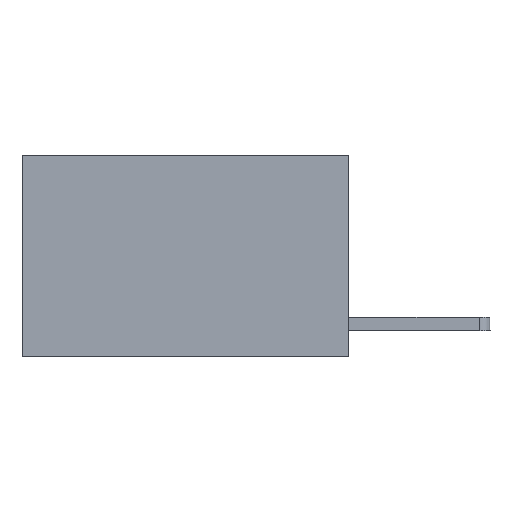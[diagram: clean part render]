
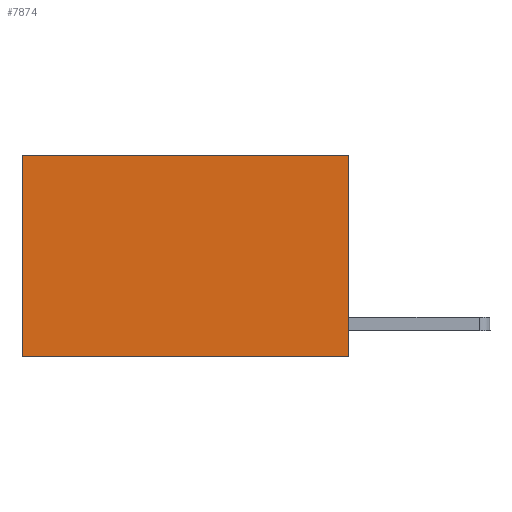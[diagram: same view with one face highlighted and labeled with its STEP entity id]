
A CAD part, left-side view. The second image highlights one B-rep face of the part: STEP entity #7874.
In plain terms, the highlighted planar face has unit normal (-1, 0, 0).
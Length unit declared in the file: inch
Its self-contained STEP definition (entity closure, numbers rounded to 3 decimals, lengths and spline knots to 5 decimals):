
#74 = EDGE_CURVE ( 'NONE', #4193, #2986, #7258, .T. ) ;
#390 = DIRECTION ( 'NONE',  ( 0., 1., 0. ) ) ;
#688 = CARTESIAN_POINT ( 'NONE',  ( 0.2625, 0., 0. ) ) ;
#774 = DIRECTION ( 'NONE',  ( 0., 0., -1. ) ) ;
#802 = DIRECTION ( 'NONE',  ( 0., 0., -1. ) ) ;
#911 = VECTOR ( 'NONE', #802, 39.37008 ) ;
#1186 = CARTESIAN_POINT ( 'NONE',  ( 0.2625, 0., -0.37 ) ) ;
#1474 = CARTESIAN_POINT ( 'NONE',  ( 0.2625, 0., 0. ) ) ;
#1542 = EDGE_LOOP ( 'NONE', ( #5234, #8449, #3500, #1996 ) ) ;
#1859 = EDGE_CURVE ( 'NONE', #2853, #7615, #8200, .T. ) ;
#1996 = ORIENTED_EDGE ( 'NONE', *, *, #3103, .T. ) ;
#2069 = AXIS2_PLACEMENT_3D ( 'NONE', #6300, #4270, #774 ) ;
#2853 = VERTEX_POINT ( 'NONE', #3470 ) ;
#2986 = VERTEX_POINT ( 'NONE', #5778 ) ;
#3103 = EDGE_CURVE ( 'NONE', #2853, #4193, #7926, .T. ) ;
#3239 = VECTOR ( 'NONE', #6705, 39.37008 ) ;
#3470 = CARTESIAN_POINT ( 'NONE',  ( 0.2625, 0., 0. ) ) ;
#3500 = ORIENTED_EDGE ( 'NONE', *, *, #1859, .F. ) ;
#3734 = VECTOR ( 'NONE', #8629, 39.37008 ) ;
#4193 = VERTEX_POINT ( 'NONE', #4853 ) ;
#4270 = DIRECTION ( 'NONE',  ( 1., 0., 0. ) ) ;
#4509 = LINE ( 'NONE', #1186, #8508 ) ;
#4853 = CARTESIAN_POINT ( 'NONE',  ( 0.2625, 0.6, 0. ) ) ;
#5234 = ORIENTED_EDGE ( 'NONE', *, *, #74, .T. ) ;
#5778 = CARTESIAN_POINT ( 'NONE',  ( 0.2625, 0.6, -0.37 ) ) ;
#6005 = CARTESIAN_POINT ( 'NONE',  ( 0.2625, 0.6, 0. ) ) ;
#6300 = CARTESIAN_POINT ( 'NONE',  ( 0.2625, 0., 0. ) ) ;
#6705 = DIRECTION ( 'NONE',  ( 0., 0., -1. ) ) ;
#6825 = FACE_OUTER_BOUND ( 'NONE', #1542, .T. ) ;
#7115 = EDGE_CURVE ( 'NONE', #7615, #2986, #4509, .T. ) ;
#7258 = LINE ( 'NONE', #6005, #3239 ) ;
#7614 = PLANE ( 'NONE',  #2069 ) ;
#7615 = VERTEX_POINT ( 'NONE', #8404 ) ;
#7874 = ADVANCED_FACE ( 'NONE', ( #6825 ), #7614, .F. ) ;
#7926 = LINE ( 'NONE', #688, #3734 ) ;
#8200 = LINE ( 'NONE', #1474, #911 ) ;
#8404 = CARTESIAN_POINT ( 'NONE',  ( 0.2625, 0., -0.37 ) ) ;
#8449 = ORIENTED_EDGE ( 'NONE', *, *, #7115, .F. ) ;
#8508 = VECTOR ( 'NONE', #390, 39.37008 ) ;
#8629 = DIRECTION ( 'NONE',  ( 0., 1., 0. ) ) ;
